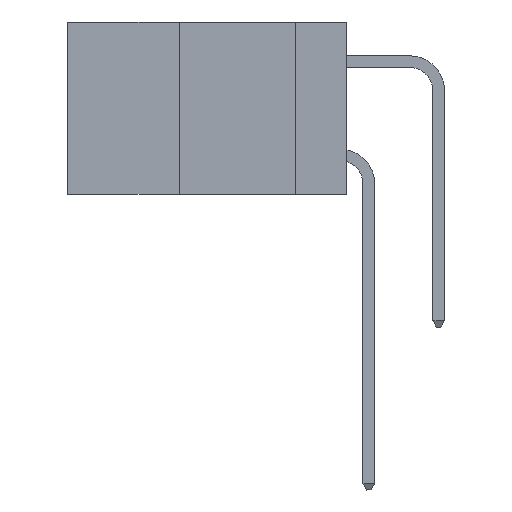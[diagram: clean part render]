
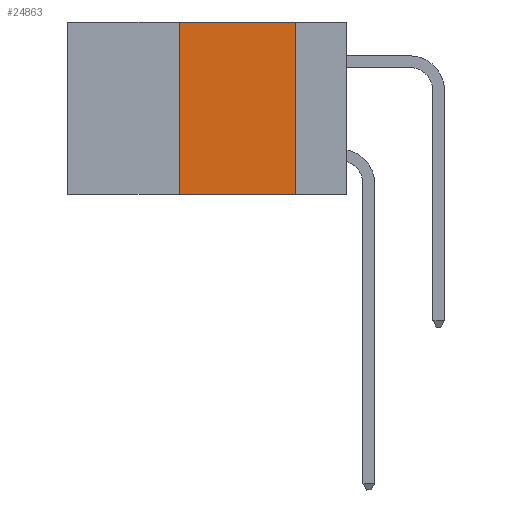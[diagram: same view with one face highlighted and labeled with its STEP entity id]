
A CAD part, left-side view. The second image highlights one B-rep face of the part: STEP entity #24863.
In plain terms, the highlighted planar face has unit normal (-1, 0, 0).
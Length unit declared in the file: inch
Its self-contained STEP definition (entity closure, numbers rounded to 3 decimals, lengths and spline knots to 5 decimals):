
#1954 = ORIENTED_EDGE ( 'NONE', *, *, #11614, .F. ) ;
#2276 = PLANE ( 'NONE',  #14352 ) ;
#2419 = DIRECTION ( 'NONE',  ( 0., 0., 1. ) ) ;
#2571 = VERTEX_POINT ( 'NONE', #7730 ) ;
#6763 = CARTESIAN_POINT ( 'NONE',  ( 0., 0.36, 0. ) ) ;
#7031 = CARTESIAN_POINT ( 'NONE',  ( 0., 0.36, -0.37 ) ) ;
#7730 = CARTESIAN_POINT ( 'NONE',  ( 0., 0.11, -0.37 ) ) ;
#8426 = DIRECTION ( 'NONE',  ( 0., -1., 0. ) ) ;
#8503 = DIRECTION ( 'NONE',  ( 1., 0., 0. ) ) ;
#8529 = VECTOR ( 'NONE', #2419, 39.37008 ) ;
#10040 = VECTOR ( 'NONE', #11968, 39.37008 ) ;
#10463 = CARTESIAN_POINT ( 'NONE',  ( 0., 0.6, -0.37 ) ) ;
#10539 = CARTESIAN_POINT ( 'NONE',  ( 0., 0.36, 0. ) ) ;
#11614 = EDGE_CURVE ( 'NONE', #15994, #16619, #15896, .T. ) ;
#11916 = EDGE_CURVE ( 'NONE', #16619, #2571, #13055, .T. ) ;
#11968 = DIRECTION ( 'NONE',  ( 0., -1., 0. ) ) ;
#12410 = CARTESIAN_POINT ( 'NONE',  ( 0., 0.11, 0. ) ) ;
#12580 = FACE_OUTER_BOUND ( 'NONE', #24540, .T. ) ;
#13055 = LINE ( 'NONE', #19422, #16968 ) ;
#14352 = AXIS2_PLACEMENT_3D ( 'NONE', #18538, #8503, #14605 ) ;
#14605 = DIRECTION ( 'NONE',  ( 0., 0., -1. ) ) ;
#15896 = LINE ( 'NONE', #18341, #10040 ) ;
#15994 = VERTEX_POINT ( 'NONE', #10539 ) ;
#16619 = VERTEX_POINT ( 'NONE', #12410 ) ;
#16793 = LINE ( 'NONE', #6763, #8529 ) ;
#16833 = LINE ( 'NONE', #10463, #19101 ) ;
#16968 = VECTOR ( 'NONE', #21326, 39.37008 ) ;
#18122 = EDGE_CURVE ( 'NONE', #18281, #15994, #16793, .T. ) ;
#18281 = VERTEX_POINT ( 'NONE', #7031 ) ;
#18341 = CARTESIAN_POINT ( 'NONE',  ( 0., 0.6, 0. ) ) ;
#18538 = CARTESIAN_POINT ( 'NONE',  ( 0., 0.6, 0. ) ) ;
#19101 = VECTOR ( 'NONE', #8426, 39.37008 ) ;
#19422 = CARTESIAN_POINT ( 'NONE',  ( 0., 0.11, 0. ) ) ;
#21326 = DIRECTION ( 'NONE',  ( 0., 0., -1. ) ) ;
#21739 = ORIENTED_EDGE ( 'NONE', *, *, #11916, .F. ) ;
#22420 = ORIENTED_EDGE ( 'NONE', *, *, #18122, .F. ) ;
#24131 = EDGE_CURVE ( 'NONE', #18281, #2571, #16833, .T. ) ;
#24540 = EDGE_LOOP ( 'NONE', ( #21739, #1954, #22420, #25403 ) ) ;
#24863 = ADVANCED_FACE ( 'NONE', ( #12580 ), #2276, .F. ) ;
#25403 = ORIENTED_EDGE ( 'NONE', *, *, #24131, .T. ) ;
